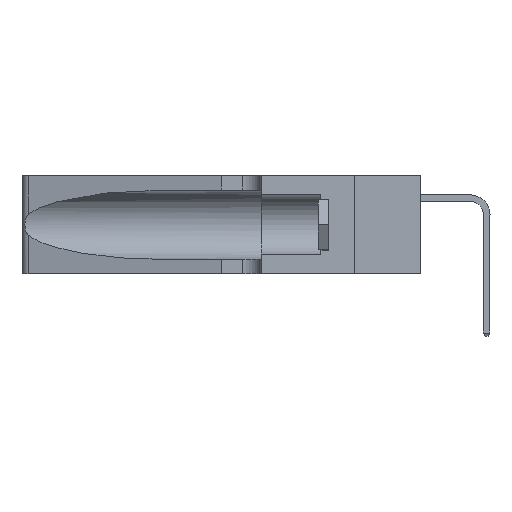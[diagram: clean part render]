
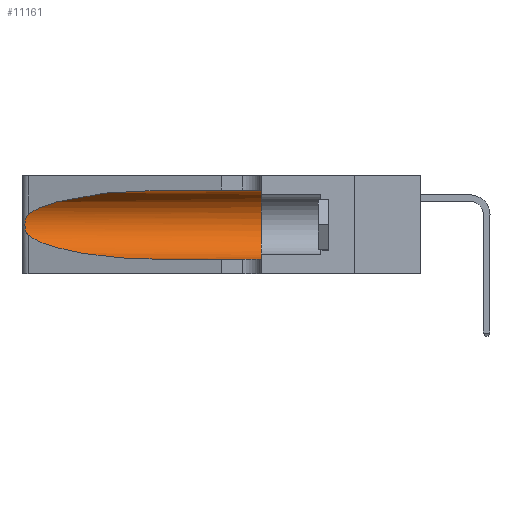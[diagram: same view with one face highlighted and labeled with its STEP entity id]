
A CAD part, left-side view. The second image highlights one B-rep face of the part: STEP entity #11161.
In plain terms, the highlighted cylindrical face has radius 3.308 mm (diameter 6.617 mm), a partial arc.
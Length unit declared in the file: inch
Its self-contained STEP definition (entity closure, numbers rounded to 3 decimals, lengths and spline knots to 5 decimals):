
#245 = CARTESIAN_POINT ( 'NONE',  ( 0.25487, 1.22718, 0.14631 ) ) ;
#268 = EDGE_CURVE ( 'NONE', #6493, #17947, #21277, .T. ) ;
#1511 = CARTESIAN_POINT ( 'NONE',  ( 0.26075, 1.23896, 0.19203 ) ) ;
#1680 = B_SPLINE_CURVE_WITH_KNOTS ( 'NONE', 3,
 ( #9190, #11817, #29668, #14421, #32242, #16984, #1511, #19568, #4110, #22101, #6687, #24664, #9298, #27239 ),
 .UNSPECIFIED., .F., .F.,
 ( 4, 2, 2, 2, 2, 2, 4 ),
 ( 0., 0.00027, 0.00053, 0.00107, 0.0016, 0.00187, 0.00214 ),
 .UNSPECIFIED. ) ;
#2712 = CIRCLE ( 'NONE', #31876, 0.13025 ) ;
#2848 = CARTESIAN_POINT ( 'NONE',  ( 0.18966, 0.96281, 0.05475 ) ) ;
#4110 = CARTESIAN_POINT ( 'NONE',  ( 0.26017, 1.23833, 0.17102 ) ) ;
#4348 = LINE ( 'NONE', #25151, #22467 ) ;
#4693 = DIRECTION ( 'NONE',  ( 0., -1., 0. ) ) ;
#5114 = AXIS2_PLACEMENT_3D ( 'NONE', #23499, #13244, #20830 ) ;
#5230 = FACE_OUTER_BOUND ( 'NONE', #32864, .T. ) ;
#6493 = VERTEX_POINT ( 'NONE', #19482 ) ;
#6525 = CARTESIAN_POINT ( 'NONE',  ( 0.1305, 1.61858, 0.05475 ) ) ;
#6687 = CARTESIAN_POINT ( 'NONE',  ( 0.25789, 1.23486, 0.15765 ) ) ;
#6848 = CARTESIAN_POINT ( 'NONE',  ( 0.1305, 0.72297, 0.31525 ) ) ;
#7599 = VECTOR ( 'NONE', #16929, 39.37008 ) ;
#7623 = CARTESIAN_POINT ( 'NONE',  ( 0.1305, 0.35, 0.31525 ) ) ;
#8949 = CARTESIAN_POINT ( 'NONE',  ( 0.1305, 0.35, 0.05475 ) ) ;
#9190 = CARTESIAN_POINT ( 'NONE',  ( 0.25487, 1.22718, 0.22369 ) ) ;
#9298 = CARTESIAN_POINT ( 'NONE',  ( 0.25555, 1.22993, 0.14849 ) ) ;
#10403 = ORIENTED_EDGE ( 'NONE', *, *, #13596, .F. ) ;
#11161 = ADVANCED_FACE ( 'NONE', ( #5230 ), #11333, .F. ) ;
#11333 = CYLINDRICAL_SURFACE ( 'NONE', #5114, 0.13025 ) ;
#11371 =( BOUNDED_CURVE ( )  B_SPLINE_CURVE ( 3, ( #6848, #19725, #29939, #14681 ),
 .UNSPECIFIED., .F., .T. ) 
 B_SPLINE_CURVE_WITH_KNOTS ( ( 4, 4 ),
 ( 1.5708, 2.84003 ),
 .UNSPECIFIED. ) 
 CURVE ( )  GEOMETRIC_REPRESENTATION_ITEM ( )  RATIONAL_B_SPLINE_CURVE ( ( 1., 0.87, 0.87, 1. ) ) 
 REPRESENTATION_ITEM ( '' )  );
#11717 = VERTEX_POINT ( 'NONE', #7623 ) ;
#11817 = CARTESIAN_POINT ( 'NONE',  ( 0.25555, 1.22994, 0.2215 ) ) ;
#12515 = EDGE_CURVE ( 'NONE', #25721, #6493, #19262, .T. ) ;
#12556 = EDGE_CURVE ( 'NONE', #11717, #17947, #2712, .T. ) ;
#13244 = DIRECTION ( 'NONE',  ( 0., -1., 0. ) ) ;
#13507 = DIRECTION ( 'NONE',  ( 0., 1., 0. ) ) ;
#13596 = EDGE_CURVE ( 'NONE', #14686, #11717, #4348, .T. ) ;
#14421 = CARTESIAN_POINT ( 'NONE',  ( 0.25787, 1.23484, 0.2124 ) ) ;
#14681 = CARTESIAN_POINT ( 'NONE',  ( 0.25487, 1.22718, 0.22369 ) ) ;
#14686 = VERTEX_POINT ( 'NONE', #19879 ) ;
#15460 = ORIENTED_EDGE ( 'NONE', *, *, #12556, .F. ) ;
#16501 = CARTESIAN_POINT ( 'NONE',  ( 0.25487, 1.22718, 0.22369 ) ) ;
#16929 = DIRECTION ( 'NONE',  ( 0., -1., 0. ) ) ;
#16984 = CARTESIAN_POINT ( 'NONE',  ( 0.26018, 1.23835, 0.19895 ) ) ;
#17266 = EDGE_CURVE ( 'NONE', #14686, #17912, #11371, .T. ) ;
#17912 = VERTEX_POINT ( 'NONE', #16501 ) ;
#17947 = VERTEX_POINT ( 'NONE', #8949 ) ;
#18885 = CARTESIAN_POINT ( 'NONE',  ( 0.25487, 1.22718, 0.14631 ) ) ;
#19262 =( BOUNDED_CURVE ( )  B_SPLINE_CURVE ( 3, ( #245, #23327, #2848, #20880 ),
 .UNSPECIFIED., .F., .F. ) 
 B_SPLINE_CURVE_WITH_KNOTS ( ( 4, 4 ),
 ( 3.44316, 4.71239 ),
 .UNSPECIFIED. ) 
 CURVE ( )  GEOMETRIC_REPRESENTATION_ITEM ( )  RATIONAL_B_SPLINE_CURVE ( ( 1., 0.87, 0.87, 1. ) ) 
 REPRESENTATION_ITEM ( '' )  );
#19273 = EDGE_CURVE ( 'NONE', #17912, #25721, #1680, .T. ) ;
#19482 = CARTESIAN_POINT ( 'NONE',  ( 0.1305, 0.72297, 0.05475 ) ) ;
#19568 = CARTESIAN_POINT ( 'NONE',  ( 0.26075, 1.23896, 0.178 ) ) ;
#19725 = CARTESIAN_POINT ( 'NONE',  ( 0.18966, 0.96281, 0.31525 ) ) ;
#19879 = CARTESIAN_POINT ( 'NONE',  ( 0.1305, 0.72297, 0.31525 ) ) ;
#20830 = DIRECTION ( 'NONE',  ( 0., 0., -1. ) ) ;
#20880 = CARTESIAN_POINT ( 'NONE',  ( 0.1305, 0.72297, 0.05475 ) ) ;
#21277 = LINE ( 'NONE', #6525, #7599 ) ;
#22101 = CARTESIAN_POINT ( 'NONE',  ( 0.25856, 1.23593, 0.16098 ) ) ;
#22467 = VECTOR ( 'NONE', #4693, 39.37008 ) ;
#22898 = ORIENTED_EDGE ( 'NONE', *, *, #17266, .T. ) ;
#23112 = ORIENTED_EDGE ( 'NONE', *, *, #268, .T. ) ;
#23327 = CARTESIAN_POINT ( 'NONE',  ( 0.2373, 1.15595, 0.08982 ) ) ;
#23403 = ORIENTED_EDGE ( 'NONE', *, *, #12515, .T. ) ;
#23499 = CARTESIAN_POINT ( 'NONE',  ( 0.1305, 1.61858, 0.185 ) ) ;
#24664 = CARTESIAN_POINT ( 'NONE',  ( 0.25639, 1.23186, 0.15144 ) ) ;
#25151 = CARTESIAN_POINT ( 'NONE',  ( 0.1305, 1.61858, 0.31525 ) ) ;
#25721 = VERTEX_POINT ( 'NONE', #18885 ) ;
#27239 = CARTESIAN_POINT ( 'NONE',  ( 0.25487, 1.22718, 0.14631 ) ) ;
#28778 = CARTESIAN_POINT ( 'NONE',  ( 0.1305, 0.35, 0.185 ) ) ;
#29668 = CARTESIAN_POINT ( 'NONE',  ( 0.25639, 1.23184, 0.21858 ) ) ;
#29939 = CARTESIAN_POINT ( 'NONE',  ( 0.2373, 1.15595, 0.28018 ) ) ;
#31344 = DIRECTION ( 'NONE',  ( 0., 0., 1. ) ) ;
#31876 = AXIS2_PLACEMENT_3D ( 'NONE', #28778, #13507, #31344 ) ;
#32044 = ORIENTED_EDGE ( 'NONE', *, *, #19273, .T. ) ;
#32242 = CARTESIAN_POINT ( 'NONE',  ( 0.25854, 1.2359, 0.20912 ) ) ;
#32864 = EDGE_LOOP ( 'NONE', ( #22898, #32044, #23403, #23112, #15460, #10403 ) ) ;
